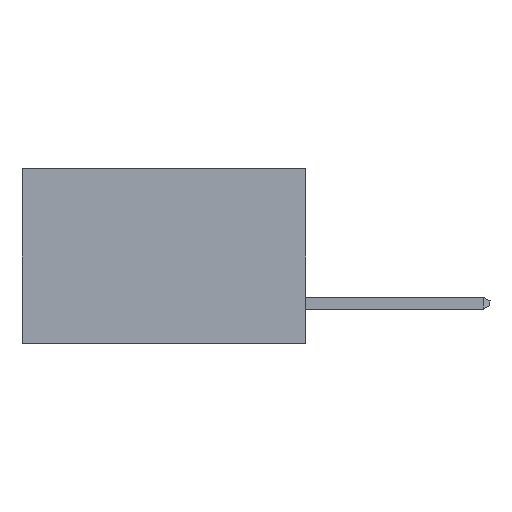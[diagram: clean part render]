
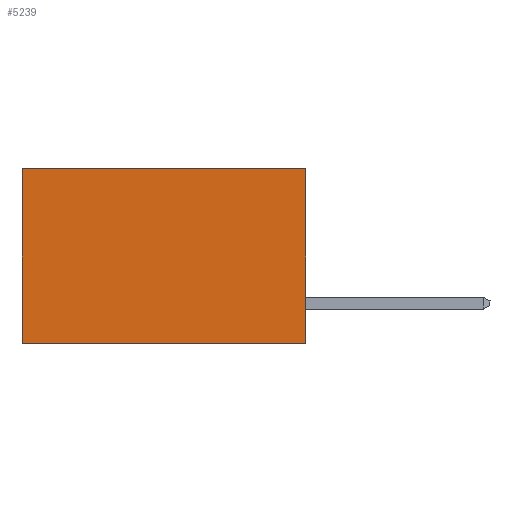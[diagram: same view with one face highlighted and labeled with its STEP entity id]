
A CAD part, left-side view. The second image highlights one B-rep face of the part: STEP entity #5239.
In plain terms, the highlighted planar face has unit normal (-1, 0, 0).
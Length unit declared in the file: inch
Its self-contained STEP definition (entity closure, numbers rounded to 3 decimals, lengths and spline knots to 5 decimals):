
#385 = LINE ( 'NONE', #9105, #9627 ) ;
#662 = AXIS2_PLACEMENT_3D ( 'NONE', #1772, #8250, #1722 ) ;
#736 = LINE ( 'NONE', #3335, #4554 ) ;
#824 = CARTESIAN_POINT ( 'NONE',  ( 0.2615, 0.6, -0.37 ) ) ;
#1019 = ORIENTED_EDGE ( 'NONE', *, *, #3030, .F. ) ;
#1162 = DIRECTION ( 'NONE',  ( 0., 0., -1. ) ) ;
#1197 = CARTESIAN_POINT ( 'NONE',  ( 0.2615, 0.6, 0. ) ) ;
#1722 = DIRECTION ( 'NONE',  ( 0., 0., -1. ) ) ;
#1772 = CARTESIAN_POINT ( 'NONE',  ( 0.2615, 0., -0.37 ) ) ;
#1885 = CARTESIAN_POINT ( 'NONE',  ( 0.2615, 0., 0. ) ) ;
#2356 = ORIENTED_EDGE ( 'NONE', *, *, #4043, .T. ) ;
#2515 = EDGE_LOOP ( 'NONE', ( #6619, #1019, #8000, #2356 ) ) ;
#2621 = EDGE_CURVE ( 'NONE', #5367, #3846, #385, .T. ) ;
#3030 = EDGE_CURVE ( 'NONE', #3846, #6045, #6582, .T. ) ;
#3335 = CARTESIAN_POINT ( 'NONE',  ( 0.2615, 0., 0. ) ) ;
#3428 = LINE ( 'NONE', #824, #5080 ) ;
#3846 = VERTEX_POINT ( 'NONE', #6760 ) ;
#4043 = EDGE_CURVE ( 'NONE', #5367, #7093, #736, .T. ) ;
#4554 = VECTOR ( 'NONE', #4827, 39.37008 ) ;
#4827 = DIRECTION ( 'NONE',  ( 0., 1., 0. ) ) ;
#5080 = VECTOR ( 'NONE', #7328, 39.37008 ) ;
#5084 = PLANE ( 'NONE',  #662 ) ;
#5239 = ADVANCED_FACE ( 'NONE', ( #6640 ), #5084, .F. ) ;
#5367 = VERTEX_POINT ( 'NONE', #1885 ) ;
#5385 = CARTESIAN_POINT ( 'NONE',  ( 0.2615, 0.6, -0.37 ) ) ;
#5662 = EDGE_CURVE ( 'NONE', #7093, #6045, #3428, .T. ) ;
#5728 = VECTOR ( 'NONE', #5895, 39.37008 ) ;
#5895 = DIRECTION ( 'NONE',  ( 0., 1., 0. ) ) ;
#5950 = CARTESIAN_POINT ( 'NONE',  ( 0.2615, 0., -0.37 ) ) ;
#6045 = VERTEX_POINT ( 'NONE', #5385 ) ;
#6582 = LINE ( 'NONE', #5950, #5728 ) ;
#6619 = ORIENTED_EDGE ( 'NONE', *, *, #5662, .T. ) ;
#6640 = FACE_OUTER_BOUND ( 'NONE', #2515, .T. ) ;
#6760 = CARTESIAN_POINT ( 'NONE',  ( 0.2615, 0., -0.37 ) ) ;
#7093 = VERTEX_POINT ( 'NONE', #1197 ) ;
#7328 = DIRECTION ( 'NONE',  ( 0., 0., -1. ) ) ;
#8000 = ORIENTED_EDGE ( 'NONE', *, *, #2621, .F. ) ;
#8250 = DIRECTION ( 'NONE',  ( 1., 0., 0. ) ) ;
#9105 = CARTESIAN_POINT ( 'NONE',  ( 0.2615, 0., -0.37 ) ) ;
#9627 = VECTOR ( 'NONE', #1162, 39.37008 ) ;
